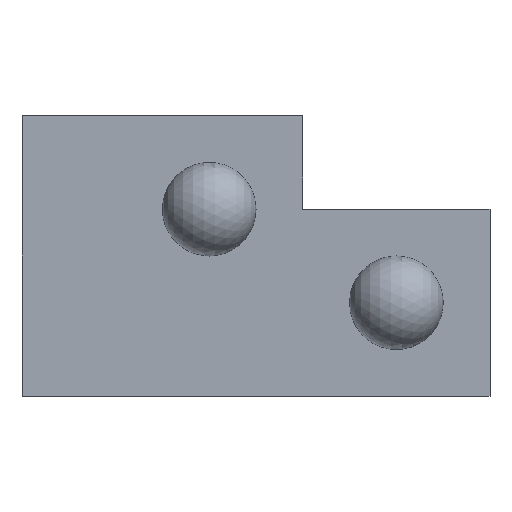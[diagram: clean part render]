
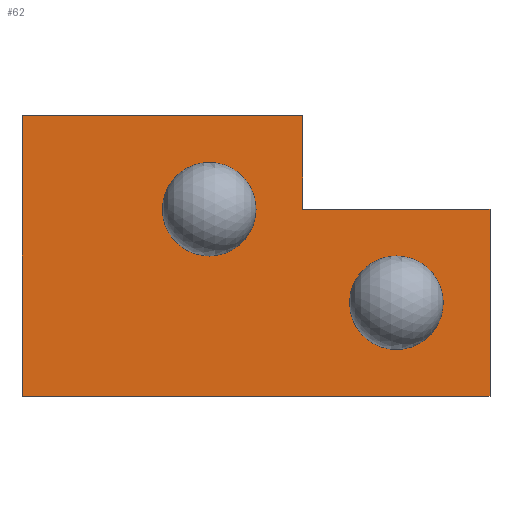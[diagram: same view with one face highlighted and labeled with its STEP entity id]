
A CAD part, left-side view. The second image highlights one B-rep face of the part: STEP entity #62.
In plain terms, the highlighted planar face has unit normal (-1, 0, 0).
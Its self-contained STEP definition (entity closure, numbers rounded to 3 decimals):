
#4 = CARTESIAN_POINT ( 'NONE',  ( 0., 10., -10. ) ) ;
#16 = CARTESIAN_POINT ( 'NONE',  ( 0., 0., 0. ) ) ;
#21 = AXIS2_PLACEMENT_3D ( 'NONE', #463, #113, #506 ) ;
#37 = VECTOR ( 'NONE', #194, 1000. ) ;
#46 = FACE_OUTER_BOUND ( 'NONE', #656, .T. ) ;
#52 = CARTESIAN_POINT ( 'NONE',  ( 0., -15., -10. ) ) ;
#62 = ADVANCED_FACE ( 'NONE', ( #130, #46, #690 ), #606, .F. ) ;
#64 = CARTESIAN_POINT ( 'NONE',  ( 0., 0., 5. ) ) ;
#99 = EDGE_CURVE ( 'NONE', #242, #380, #687, .T. ) ;
#113 = DIRECTION ( 'NONE',  ( -1., 0., 0. ) ) ;
#115 = CARTESIAN_POINT ( 'NONE',  ( 0., -10., -7.5 ) ) ;
#122 = DIRECTION ( 'NONE',  ( 0., 0., -1. ) ) ;
#130 = FACE_BOUND ( 'NONE', #706, .T. ) ;
#161 = LINE ( 'NONE', #563, #694 ) ;
#171 = CARTESIAN_POINT ( 'NONE',  ( 0., -10., -2.5 ) ) ;
#178 = CARTESIAN_POINT ( 'NONE',  ( 0., -5., 0. ) ) ;
#184 = LINE ( 'NONE', #185, #332 ) ;
#185 = CARTESIAN_POINT ( 'NONE',  ( 0., 5., -10. ) ) ;
#190 = DIRECTION ( 'NONE',  ( -1., 0., 0. ) ) ;
#192 = CARTESIAN_POINT ( 'NONE',  ( 0., -15., 0. ) ) ;
#194 = DIRECTION ( 'NONE',  ( 0., 0., -1. ) ) ;
#200 = EDGE_LOOP ( 'NONE', ( #576, #679 ) ) ;
#215 = VERTEX_POINT ( 'NONE', #178 ) ;
#242 = VERTEX_POINT ( 'NONE', #171 ) ;
#244 = CARTESIAN_POINT ( 'NONE',  ( 0., 0., 2.5 ) ) ;
#258 = DIRECTION ( 'NONE',  ( 0., 0., 1. ) ) ;
#269 = AXIS2_PLACEMENT_3D ( 'NONE', #625, #367, #336 ) ;
#297 = EDGE_CURVE ( 'NONE', #620, #634, #445, .T. ) ;
#306 = EDGE_CURVE ( 'NONE', #634, #620, #446, .T. ) ;
#310 = VERTEX_POINT ( 'NONE', #4 ) ;
#311 = EDGE_CURVE ( 'NONE', #350, #342, #430, .T. ) ;
#317 = EDGE_CURVE ( 'NONE', #310, #350, #452, .T. ) ;
#325 = DIRECTION ( 'NONE',  ( 0., 1., 0. ) ) ;
#328 = EDGE_CURVE ( 'NONE', #526, #310, #184, .T. ) ;
#329 = ORIENTED_EDGE ( 'NONE', *, *, #348, .F. ) ;
#332 = VECTOR ( 'NONE', #660, 1000. ) ;
#336 = DIRECTION ( 'NONE',  ( 0., 0., -1. ) ) ;
#341 = ORIENTED_EDGE ( 'NONE', *, *, #328, .F. ) ;
#342 = VERTEX_POINT ( 'NONE', #616 ) ;
#348 = EDGE_CURVE ( 'NONE', #421, #526, #705, .T. ) ;
#350 = VERTEX_POINT ( 'NONE', #509 ) ;
#352 = EDGE_CURVE ( 'NONE', #421, #215, #161, .T. ) ;
#356 = EDGE_CURVE ( 'NONE', #342, #215, #431, .T. ) ;
#366 = CARTESIAN_POINT ( 'NONE',  ( 0., -15., -10. ) ) ;
#367 = DIRECTION ( 'NONE',  ( -1., 0., 0. ) ) ;
#368 = EDGE_CURVE ( 'NONE', #380, #242, #441, .T. ) ;
#371 = CARTESIAN_POINT ( 'NONE',  ( 0., 0., -2.5 ) ) ;
#379 = DIRECTION ( 'NONE',  ( -1., 0., 0. ) ) ;
#380 = VERTEX_POINT ( 'NONE', #115 ) ;
#388 = ORIENTED_EDGE ( 'NONE', *, *, #317, .F. ) ;
#406 = ORIENTED_EDGE ( 'NONE', *, *, #352, .T. ) ;
#414 = AXIS2_PLACEMENT_3D ( 'NONE', #659, #379, #712 ) ;
#421 = VERTEX_POINT ( 'NONE', #192 ) ;
#422 = AXIS2_PLACEMENT_3D ( 'NONE', #507, #190, #555 ) ;
#424 = CARTESIAN_POINT ( 'NONE',  ( 0., 10., -10. ) ) ;
#430 = LINE ( 'NONE', #64, #435 ) ;
#431 = LINE ( 'NONE', #666, #436 ) ;
#435 = VECTOR ( 'NONE', #554, 1000. ) ;
#436 = VECTOR ( 'NONE', #122, 1000. ) ;
#441 = CIRCLE ( 'NONE', #422, 2.5 ) ;
#444 = VECTOR ( 'NONE', #258, 1000. ) ;
#445 = CIRCLE ( 'NONE', #414, 2.5 ) ;
#446 = CIRCLE ( 'NONE', #21, 2.5 ) ;
#452 = LINE ( 'NONE', #424, #444 ) ;
#463 = CARTESIAN_POINT ( 'NONE',  ( 0., 0., 0. ) ) ;
#478 = DIRECTION ( 'NONE',  ( 1., 0., 0. ) ) ;
#493 = ORIENTED_EDGE ( 'NONE', *, *, #311, .F. ) ;
#506 = DIRECTION ( 'NONE',  ( 0., 0., -1. ) ) ;
#507 = CARTESIAN_POINT ( 'NONE',  ( 0., -10., -5. ) ) ;
#509 = CARTESIAN_POINT ( 'NONE',  ( 0., 10., 5. ) ) ;
#514 = ORIENTED_EDGE ( 'NONE', *, *, #356, .F. ) ;
#526 = VERTEX_POINT ( 'NONE', #366 ) ;
#534 = ORIENTED_EDGE ( 'NONE', *, *, #306, .F. ) ;
#540 = ORIENTED_EDGE ( 'NONE', *, *, #297, .F. ) ;
#554 = DIRECTION ( 'NONE',  ( 0., -1., 0. ) ) ;
#555 = DIRECTION ( 'NONE',  ( 0., 0., -1. ) ) ;
#563 = CARTESIAN_POINT ( 'NONE',  ( 0., -15., 0. ) ) ;
#576 = ORIENTED_EDGE ( 'NONE', *, *, #368, .F. ) ;
#606 = PLANE ( 'NONE',  #709 ) ;
#616 = CARTESIAN_POINT ( 'NONE',  ( 0., -5., 5. ) ) ;
#617 = DIRECTION ( 'NONE',  ( 0., 0., -1. ) ) ;
#620 = VERTEX_POINT ( 'NONE', #371 ) ;
#625 = CARTESIAN_POINT ( 'NONE',  ( 0., -10., -5. ) ) ;
#634 = VERTEX_POINT ( 'NONE', #244 ) ;
#656 = EDGE_LOOP ( 'NONE', ( #493, #388, #341, #329, #406, #514 ) ) ;
#659 = CARTESIAN_POINT ( 'NONE',  ( 0., 0., 0. ) ) ;
#660 = DIRECTION ( 'NONE',  ( 0., 1., 0. ) ) ;
#666 = CARTESIAN_POINT ( 'NONE',  ( 0., -5., 0. ) ) ;
#679 = ORIENTED_EDGE ( 'NONE', *, *, #99, .F. ) ;
#687 = CIRCLE ( 'NONE', #269, 2.5 ) ;
#690 = FACE_BOUND ( 'NONE', #200, .T. ) ;
#694 = VECTOR ( 'NONE', #325, 1000. ) ;
#705 = LINE ( 'NONE', #52, #37 ) ;
#706 = EDGE_LOOP ( 'NONE', ( #540, #534 ) ) ;
#709 = AXIS2_PLACEMENT_3D ( 'NONE', #16, #478, #617 ) ;
#712 = DIRECTION ( 'NONE',  ( 0., 0., -1. ) ) ;
